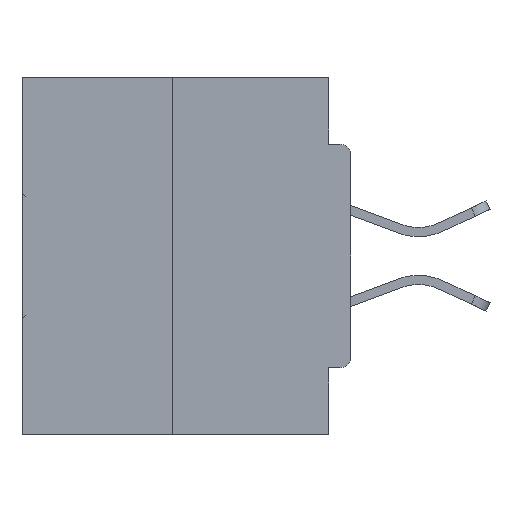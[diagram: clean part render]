
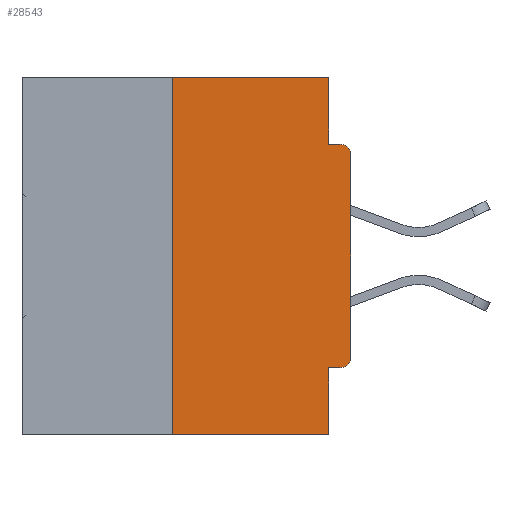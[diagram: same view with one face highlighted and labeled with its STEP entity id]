
A CAD part, left-side view. The second image highlights one B-rep face of the part: STEP entity #28543.
In plain terms, the highlighted planar face has unit normal (-1, 0, 0).
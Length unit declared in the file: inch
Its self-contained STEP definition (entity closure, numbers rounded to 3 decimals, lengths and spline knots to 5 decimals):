
#258 = VECTOR ( 'NONE', #7666, 39.37008 ) ;
#373 = DIRECTION ( 'NONE',  ( -1., 0., 0. ) ) ;
#500 = AXIS2_PLACEMENT_3D ( 'NONE', #36207, #5925, #22815 ) ;
#2142 = VECTOR ( 'NONE', #14416, 39.37008 ) ;
#2320 = EDGE_CURVE ( 'NONE', #13241, #3952, #10484, .T. ) ;
#2537 = DIRECTION ( 'NONE',  ( 0., 0., -1. ) ) ;
#3075 = EDGE_CURVE ( 'NONE', #19271, #36291, #19307, .T. ) ;
#3952 = VERTEX_POINT ( 'NONE', #24581 ) ;
#4079 = CARTESIAN_POINT ( 'NONE',  ( 0., 0., -0.4065 ) ) ;
#4599 = CARTESIAN_POINT ( 'NONE',  ( 0., 0.46, -0.5 ) ) ;
#5077 = CARTESIAN_POINT ( 'NONE',  ( 0., 0., 0. ) ) ;
#5633 = VERTEX_POINT ( 'NONE', #40795 ) ;
#5788 = CARTESIAN_POINT ( 'NONE',  ( 0., 0.031, 0. ) ) ;
#5925 = DIRECTION ( 'NONE',  ( 1., 0., 0. ) ) ;
#7194 = LINE ( 'NONE', #5077, #15657 ) ;
#7666 = DIRECTION ( 'NONE',  ( 0., 1., 0. ) ) ;
#8422 = CARTESIAN_POINT ( 'NONE',  ( 0., 0., -0.3915 ) ) ;
#8904 = CARTESIAN_POINT ( 'NONE',  ( 0., 0.25, 0. ) ) ;
#8931 = VERTEX_POINT ( 'NONE', #19966 ) ;
#9498 = PLANE ( 'NONE',  #500 ) ;
#10343 = VECTOR ( 'NONE', #36509, 39.37008 ) ;
#10484 = LINE ( 'NONE', #4599, #41627 ) ;
#11186 = CARTESIAN_POINT ( 'NONE',  ( 0., 0., -0.0935 ) ) ;
#11944 = LINE ( 'NONE', #22966, #10343 ) ;
#12389 = VERTEX_POINT ( 'NONE', #8422 ) ;
#12849 = ORIENTED_EDGE ( 'NONE', *, *, #3075, .F. ) ;
#13087 = EDGE_CURVE ( 'NONE', #5633, #8931, #21563, .T. ) ;
#13124 = VERTEX_POINT ( 'NONE', #39174 ) ;
#13241 = VERTEX_POINT ( 'NONE', #20793 ) ;
#14416 = DIRECTION ( 'NONE',  ( 0., -1., 0. ) ) ;
#14524 = ORIENTED_EDGE ( 'NONE', *, *, #2320, .T. ) ;
#14759 = AXIS2_PLACEMENT_3D ( 'NONE', #19941, #26726, #43497 ) ;
#15523 = EDGE_CURVE ( 'NONE', #19271, #12389, #28728, .T. ) ;
#15657 = VECTOR ( 'NONE', #22236, 39.37008 ) ;
#17861 = EDGE_CURVE ( 'NONE', #13241, #20733, #22306, .T. ) ;
#18238 = DIRECTION ( 'NONE',  ( 0., -1., 0. ) ) ;
#19271 = VERTEX_POINT ( 'NONE', #21918 ) ;
#19307 = LINE ( 'NONE', #4079, #258 ) ;
#19941 = CARTESIAN_POINT ( 'NONE',  ( 0., 0.015, -0.1085 ) ) ;
#19966 = CARTESIAN_POINT ( 'NONE',  ( 0., 0.031, -0.0935 ) ) ;
#20726 = ORIENTED_EDGE ( 'NONE', *, *, #34047, .F. ) ;
#20733 = VERTEX_POINT ( 'NONE', #8904 ) ;
#20793 = CARTESIAN_POINT ( 'NONE',  ( 0., 0.25, -0.5 ) ) ;
#21283 = VECTOR ( 'NONE', #43661, 39.37008 ) ;
#21563 = LINE ( 'NONE', #5788, #29428 ) ;
#21789 = CARTESIAN_POINT ( 'NONE',  ( 0., 0., -0.1085 ) ) ;
#21918 = CARTESIAN_POINT ( 'NONE',  ( 0., 0.015, -0.4065 ) ) ;
#22236 = DIRECTION ( 'NONE',  ( 0., 0., 1. ) ) ;
#22306 = LINE ( 'NONE', #36892, #21283 ) ;
#22765 = ORIENTED_EDGE ( 'NONE', *, *, #39865, .F. ) ;
#22815 = DIRECTION ( 'NONE',  ( 0., 0., -1. ) ) ;
#22966 = CARTESIAN_POINT ( 'NONE',  ( 0., 0.46, 0. ) ) ;
#23416 = DIRECTION ( 'NONE',  ( 0., 0., -1. ) ) ;
#23645 = LINE ( 'NONE', #37553, #26307 ) ;
#24341 = CARTESIAN_POINT ( 'NONE',  ( 0., 0.015, -0.3915 ) ) ;
#24372 = FACE_OUTER_BOUND ( 'NONE', #39437, .T. ) ;
#24581 = CARTESIAN_POINT ( 'NONE',  ( 0., 0.031, -0.5 ) ) ;
#24653 = VERTEX_POINT ( 'NONE', #21789 ) ;
#25091 = CIRCLE ( 'NONE', #14759, 0.015 ) ;
#26014 = ORIENTED_EDGE ( 'NONE', *, *, #13087, .F. ) ;
#26307 = VECTOR ( 'NONE', #23416, 39.37008 ) ;
#26402 = CARTESIAN_POINT ( 'NONE',  ( 0., 0.031, -0.4065 ) ) ;
#26726 = DIRECTION ( 'NONE',  ( -1., 0., 0. ) ) ;
#28543 = ADVANCED_FACE ( 'NONE', ( #24372 ), #9498, .F. ) ;
#28728 = CIRCLE ( 'NONE', #38366, 0.015 ) ;
#29428 = VECTOR ( 'NONE', #2537, 39.37008 ) ;
#30810 = EDGE_CURVE ( 'NONE', #36291, #3952, #23645, .T. ) ;
#30954 = ORIENTED_EDGE ( 'NONE', *, *, #31521, .T. ) ;
#31425 = ORIENTED_EDGE ( 'NONE', *, *, #15523, .T. ) ;
#31502 = ORIENTED_EDGE ( 'NONE', *, *, #30810, .F. ) ;
#31521 = EDGE_CURVE ( 'NONE', #12389, #24653, #7194, .T. ) ;
#34047 = EDGE_CURVE ( 'NONE', #8931, #13124, #35960, .T. ) ;
#34660 = ORIENTED_EDGE ( 'NONE', *, *, #41019, .T. ) ;
#35960 = LINE ( 'NONE', #11186, #2142 ) ;
#36207 = CARTESIAN_POINT ( 'NONE',  ( 0., 0.46, 0. ) ) ;
#36291 = VERTEX_POINT ( 'NONE', #26402 ) ;
#36509 = DIRECTION ( 'NONE',  ( 0., -1., 0. ) ) ;
#36892 = CARTESIAN_POINT ( 'NONE',  ( 0., 0.25, 0. ) ) ;
#37217 = ORIENTED_EDGE ( 'NONE', *, *, #17861, .F. ) ;
#37553 = CARTESIAN_POINT ( 'NONE',  ( 0., 0.031, -0.5 ) ) ;
#38366 = AXIS2_PLACEMENT_3D ( 'NONE', #24341, #373, #41258 ) ;
#39174 = CARTESIAN_POINT ( 'NONE',  ( 0., 0.015, -0.0935 ) ) ;
#39437 = EDGE_LOOP ( 'NONE', ( #22765, #37217, #14524, #31502, #12849, #31425, #30954, #34660, #20726, #26014 ) ) ;
#39865 = EDGE_CURVE ( 'NONE', #20733, #5633, #11944, .T. ) ;
#40795 = CARTESIAN_POINT ( 'NONE',  ( 0., 0.031, 0. ) ) ;
#41019 = EDGE_CURVE ( 'NONE', #24653, #13124, #25091, .T. ) ;
#41258 = DIRECTION ( 'NONE',  ( 0., 0., -1. ) ) ;
#41627 = VECTOR ( 'NONE', #18238, 39.37008 ) ;
#43497 = DIRECTION ( 'NONE',  ( 0., 0., -1. ) ) ;
#43661 = DIRECTION ( 'NONE',  ( 0., 0., 1. ) ) ;
